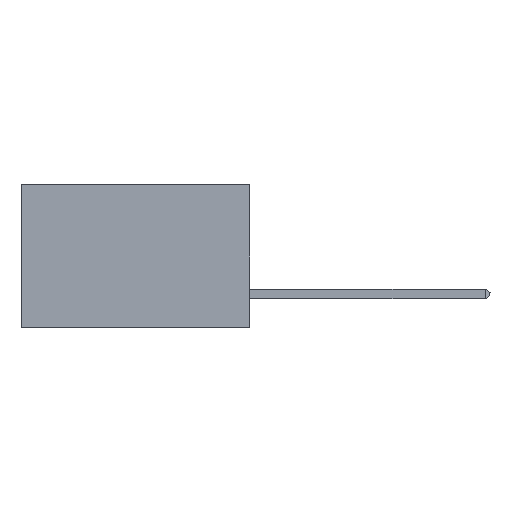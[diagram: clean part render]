
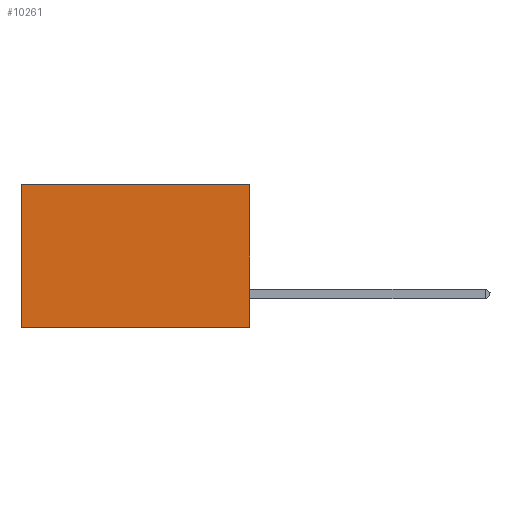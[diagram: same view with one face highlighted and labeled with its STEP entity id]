
A CAD part, left-side view. The second image highlights one B-rep face of the part: STEP entity #10261.
In plain terms, the highlighted planar face has unit normal (-1, 0, 0).
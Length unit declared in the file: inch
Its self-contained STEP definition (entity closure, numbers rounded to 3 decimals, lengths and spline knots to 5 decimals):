
#51 = CARTESIAN_POINT ( 'NONE',  ( 0.2875, 0., 0. ) ) ;
#777 = VECTOR ( 'NONE', #9754, 39.37008 ) ;
#1452 = EDGE_CURVE ( 'NONE', #11951, #10924, #9004, .T. ) ;
#1487 = VECTOR ( 'NONE', #7652, 39.37008 ) ;
#1762 = CARTESIAN_POINT ( 'NONE',  ( 0.2875, 0., -0.375 ) ) ;
#2010 = ORIENTED_EDGE ( 'NONE', *, *, #5359, .T. ) ;
#2372 = ORIENTED_EDGE ( 'NONE', *, *, #5343, .F. ) ;
#2571 = LINE ( 'NONE', #5759, #777 ) ;
#2834 = CARTESIAN_POINT ( 'NONE',  ( 0.2875, 0.6, -0.375 ) ) ;
#3015 = VECTOR ( 'NONE', #12008, 39.37008 ) ;
#3368 = ORIENTED_EDGE ( 'NONE', *, *, #9938, .F. ) ;
#4435 = CARTESIAN_POINT ( 'NONE',  ( 0.2875, 0., -0.375 ) ) ;
#4762 = CARTESIAN_POINT ( 'NONE',  ( 0.2875, 0.6, -0.375 ) ) ;
#5343 = EDGE_CURVE ( 'NONE', #11951, #11594, #2571, .T. ) ;
#5359 = EDGE_CURVE ( 'NONE', #10924, #10487, #6738, .T. ) ;
#5759 = CARTESIAN_POINT ( 'NONE',  ( 0.2875, 0., -0.375 ) ) ;
#6539 = DIRECTION ( 'NONE',  ( 0., 0., -1. ) ) ;
#6699 = CARTESIAN_POINT ( 'NONE',  ( 0.2875, 0., 0. ) ) ;
#6723 = ORIENTED_EDGE ( 'NONE', *, *, #1452, .T. ) ;
#6738 = LINE ( 'NONE', #2834, #10358 ) ;
#7652 = DIRECTION ( 'NONE',  ( 0., 1., 0. ) ) ;
#7803 = CARTESIAN_POINT ( 'NONE',  ( 0.2875, 0.6, 0. ) ) ;
#9004 = LINE ( 'NONE', #51, #1487 ) ;
#9754 = DIRECTION ( 'NONE',  ( 0., 0., -1. ) ) ;
#9938 = EDGE_CURVE ( 'NONE', #11594, #10487, #11044, .T. ) ;
#10261 = ADVANCED_FACE ( 'NONE', ( #11617 ), #10586, .F. ) ;
#10358 = VECTOR ( 'NONE', #6539, 39.37008 ) ;
#10445 = DIRECTION ( 'NONE',  ( 1., 0., 0. ) ) ;
#10487 = VERTEX_POINT ( 'NONE', #4762 ) ;
#10586 = PLANE ( 'NONE',  #11361 ) ;
#10915 = CARTESIAN_POINT ( 'NONE',  ( 0.2875, 0., -0.375 ) ) ;
#10924 = VERTEX_POINT ( 'NONE', #7803 ) ;
#11044 = LINE ( 'NONE', #10915, #3015 ) ;
#11361 = AXIS2_PLACEMENT_3D ( 'NONE', #4435, #10445, #11676 ) ;
#11425 = EDGE_LOOP ( 'NONE', ( #2010, #3368, #2372, #6723 ) ) ;
#11594 = VERTEX_POINT ( 'NONE', #1762 ) ;
#11617 = FACE_OUTER_BOUND ( 'NONE', #11425, .T. ) ;
#11676 = DIRECTION ( 'NONE',  ( 0., 0., -1. ) ) ;
#11951 = VERTEX_POINT ( 'NONE', #6699 ) ;
#12008 = DIRECTION ( 'NONE',  ( 0., 1., 0. ) ) ;
